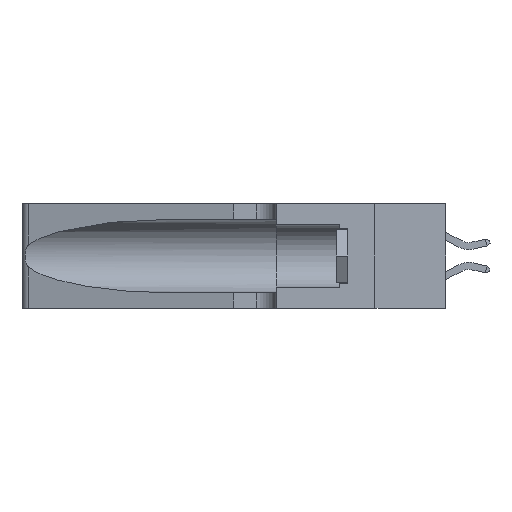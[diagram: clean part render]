
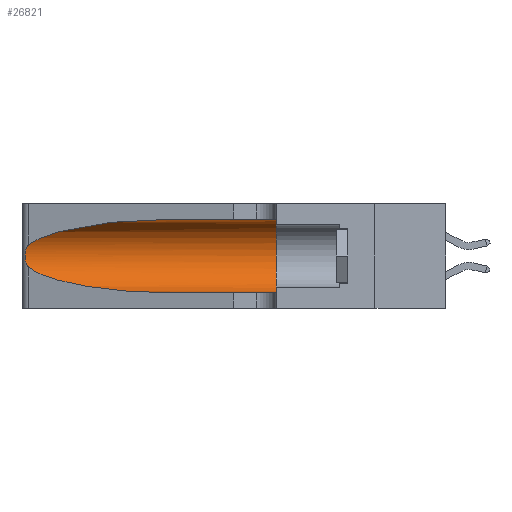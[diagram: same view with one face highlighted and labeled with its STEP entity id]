
A CAD part, left-side view. The second image highlights one B-rep face of the part: STEP entity #26821.
In plain terms, the highlighted cylindrical face has radius 3.308 mm (diameter 6.617 mm), a partial arc.
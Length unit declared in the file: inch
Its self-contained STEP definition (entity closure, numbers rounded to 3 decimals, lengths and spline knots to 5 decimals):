
#213 = EDGE_CURVE ( 'NONE', #20160, #27502, #10032, .T. ) ;
#285 = AXIS2_PLACEMENT_3D ( 'NONE', #4742, #20351, #6967 ) ;
#484 = EDGE_CURVE ( 'NONE', #13367, #15842, #21501, .T. ) ;
#1286 =( BOUNDED_CURVE ( )  B_SPLINE_CURVE ( 3, ( #19607, #17389, #21830, #8473 ),
 .UNSPECIFIED., .F., .F. ) 
 B_SPLINE_CURVE_WITH_KNOTS ( ( 4, 4 ),
 ( 1.5708, 2.84003 ),
 .UNSPECIFIED. ) 
 CURVE ( )  GEOMETRIC_REPRESENTATION_ITEM ( )  RATIONAL_B_SPLINE_CURVE ( ( 1., 0.87, 0.87, 1. ) ) 
 REPRESENTATION_ITEM ( '' )  );
#1590 = CARTESIAN_POINT ( 'NONE',  ( 0.25555, 1.22993, 0.14849 ) ) ;
#1757 = CARTESIAN_POINT ( 'NONE',  ( 0.25487, 1.22718, 0.22369 ) ) ;
#2729 = DIRECTION ( 'NONE',  ( 0., -1., 0. ) ) ;
#3697 = VECTOR ( 'NONE', #5751, 39.37008 ) ;
#3700 = EDGE_LOOP ( 'NONE', ( #7660, #9780, #17136, #18532, #4196, #22670 ) ) ;
#4055 = AXIS2_PLACEMENT_3D ( 'NONE', #13268, #11092, #24359 ) ;
#4078 = VECTOR ( 'NONE', #2729, 39.37008 ) ;
#4196 = ORIENTED_EDGE ( 'NONE', *, *, #28240, .F. ) ;
#4619 = CARTESIAN_POINT ( 'NONE',  ( 0.1305, 0.72297, 0.05475 ) ) ;
#4742 = CARTESIAN_POINT ( 'NONE',  ( 0.1305, 0.35, 0.185 ) ) ;
#5751 = DIRECTION ( 'NONE',  ( 0., -1., 0. ) ) ;
#5999 = CARTESIAN_POINT ( 'NONE',  ( 0.25787, 1.23484, 0.2124 ) ) ;
#6967 = DIRECTION ( 'NONE',  ( 0., 0., 1. ) ) ;
#7660 = ORIENTED_EDGE ( 'NONE', *, *, #16586, .T. ) ;
#7778 = EDGE_CURVE ( 'NONE', #22588, #13367, #22039, .T. ) ;
#7799 = CARTESIAN_POINT ( 'NONE',  ( 0.25487, 1.22718, 0.14631 ) ) ;
#8258 = CARTESIAN_POINT ( 'NONE',  ( 0.26018, 1.23835, 0.19895 ) ) ;
#8324 = CARTESIAN_POINT ( 'NONE',  ( 0.1305, 0.35, 0.05475 ) ) ;
#8473 = CARTESIAN_POINT ( 'NONE',  ( 0.25487, 1.22718, 0.22369 ) ) ;
#9780 = ORIENTED_EDGE ( 'NONE', *, *, #27974, .T. ) ;
#10032 = LINE ( 'NONE', #27209, #4078 ) ;
#10076 = VERTEX_POINT ( 'NONE', #1757 ) ;
#10529 = CARTESIAN_POINT ( 'NONE',  ( 0.26075, 1.23896, 0.178 ) ) ;
#10959 = FACE_OUTER_BOUND ( 'NONE', #3700, .T. ) ;
#11092 = DIRECTION ( 'NONE',  ( 0., -1., 0. ) ) ;
#12408 = CARTESIAN_POINT ( 'NONE',  ( 0.25487, 1.22718, 0.14631 ) ) ;
#12826 = CARTESIAN_POINT ( 'NONE',  ( 0.25856, 1.23593, 0.16098 ) ) ;
#13268 = CARTESIAN_POINT ( 'NONE',  ( 0.1305, 1.61858, 0.185 ) ) ;
#13323 = CARTESIAN_POINT ( 'NONE',  ( 0.1305, 0.35, 0.31525 ) ) ;
#13367 = VERTEX_POINT ( 'NONE', #4619 ) ;
#14659 = CARTESIAN_POINT ( 'NONE',  ( 0.2373, 1.15595, 0.08982 ) ) ;
#14955 = CARTESIAN_POINT ( 'NONE',  ( 0.25487, 1.22718, 0.22369 ) ) ;
#15050 = CARTESIAN_POINT ( 'NONE',  ( 0.25639, 1.23186, 0.15144 ) ) ;
#15520 = CYLINDRICAL_SURFACE ( 'NONE', #4055, 0.13025 ) ;
#15842 = VERTEX_POINT ( 'NONE', #8324 ) ;
#16118 = CARTESIAN_POINT ( 'NONE',  ( 0.1305, 1.61858, 0.05475 ) ) ;
#16586 = EDGE_CURVE ( 'NONE', #20160, #10076, #1286, .T. ) ;
#16864 = CARTESIAN_POINT ( 'NONE',  ( 0.1305, 0.72297, 0.05475 ) ) ;
#17136 = ORIENTED_EDGE ( 'NONE', *, *, #7778, .T. ) ;
#17271 = CARTESIAN_POINT ( 'NONE',  ( 0.25487, 1.22718, 0.14631 ) ) ;
#17389 = CARTESIAN_POINT ( 'NONE',  ( 0.18966, 0.96281, 0.31525 ) ) ;
#17803 = B_SPLINE_CURVE_WITH_KNOTS ( 'NONE', 3,
 ( #14955, #28148, #19404, #5999, #21605, #8258, #23826, #10529, #26030, #12826, #28246, #15050, #1590, #17271 ),
 .UNSPECIFIED., .F., .F.,
 ( 4, 2, 2, 2, 2, 2, 4 ),
 ( 0., 0.00027, 0.00053, 0.00107, 0.0016, 0.00187, 0.00214 ),
 .UNSPECIFIED. ) ;
#18532 = ORIENTED_EDGE ( 'NONE', *, *, #484, .T. ) ;
#19404 = CARTESIAN_POINT ( 'NONE',  ( 0.25639, 1.23184, 0.21858 ) ) ;
#19607 = CARTESIAN_POINT ( 'NONE',  ( 0.1305, 0.72297, 0.31525 ) ) ;
#20160 = VERTEX_POINT ( 'NONE', #23685 ) ;
#20351 = DIRECTION ( 'NONE',  ( 0., 1., 0. ) ) ;
#20621 = CIRCLE ( 'NONE', #285, 0.13025 ) ;
#21501 = LINE ( 'NONE', #16118, #3697 ) ;
#21605 = CARTESIAN_POINT ( 'NONE',  ( 0.25854, 1.2359, 0.20912 ) ) ;
#21830 = CARTESIAN_POINT ( 'NONE',  ( 0.2373, 1.15595, 0.28018 ) ) ;
#22039 =( BOUNDED_CURVE ( )  B_SPLINE_CURVE ( 3, ( #12408, #14659, #27851, #16864 ),
 .UNSPECIFIED., .F., .F. ) 
 B_SPLINE_CURVE_WITH_KNOTS ( ( 4, 4 ),
 ( 3.44316, 4.71239 ),
 .UNSPECIFIED. ) 
 CURVE ( )  GEOMETRIC_REPRESENTATION_ITEM ( )  RATIONAL_B_SPLINE_CURVE ( ( 1., 0.87, 0.87, 1. ) ) 
 REPRESENTATION_ITEM ( '' )  );
#22588 = VERTEX_POINT ( 'NONE', #7799 ) ;
#22670 = ORIENTED_EDGE ( 'NONE', *, *, #213, .F. ) ;
#23685 = CARTESIAN_POINT ( 'NONE',  ( 0.1305, 0.72297, 0.31525 ) ) ;
#23826 = CARTESIAN_POINT ( 'NONE',  ( 0.26075, 1.23896, 0.19203 ) ) ;
#24359 = DIRECTION ( 'NONE',  ( 0., 0., -1. ) ) ;
#26030 = CARTESIAN_POINT ( 'NONE',  ( 0.26017, 1.23833, 0.17102 ) ) ;
#26821 = ADVANCED_FACE ( 'NONE', ( #10959 ), #15520, .F. ) ;
#27209 = CARTESIAN_POINT ( 'NONE',  ( 0.1305, 1.61858, 0.31525 ) ) ;
#27502 = VERTEX_POINT ( 'NONE', #13323 ) ;
#27851 = CARTESIAN_POINT ( 'NONE',  ( 0.18966, 0.96281, 0.05475 ) ) ;
#27974 = EDGE_CURVE ( 'NONE', #10076, #22588, #17803, .T. ) ;
#28148 = CARTESIAN_POINT ( 'NONE',  ( 0.25555, 1.22994, 0.2215 ) ) ;
#28240 = EDGE_CURVE ( 'NONE', #27502, #15842, #20621, .T. ) ;
#28246 = CARTESIAN_POINT ( 'NONE',  ( 0.25789, 1.23486, 0.15765 ) ) ;
